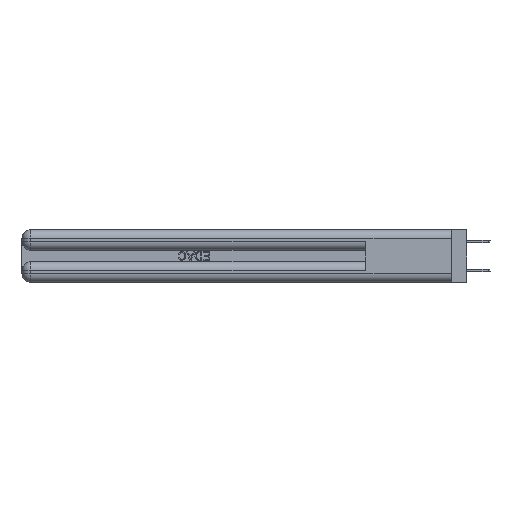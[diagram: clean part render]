
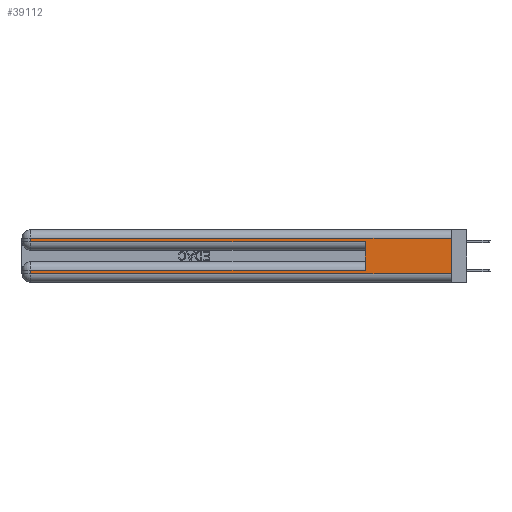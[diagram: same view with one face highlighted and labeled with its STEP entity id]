
A CAD part, left-side view. The second image highlights one B-rep face of the part: STEP entity #39112.
In plain terms, the highlighted planar face has unit normal (-1, 0, 0).
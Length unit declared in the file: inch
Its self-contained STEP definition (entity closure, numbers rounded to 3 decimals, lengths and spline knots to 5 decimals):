
#797 = CARTESIAN_POINT ( 'NONE',  ( 0., 0.6, 0.285 ) ) ;
#1355 = VECTOR ( 'NONE', #39381, 39.37008 ) ;
#1964 = VERTEX_POINT ( 'NONE', #797 ) ;
#2108 = EDGE_CURVE ( 'NONE', #13779, #41436, #46561, .T. ) ;
#2115 = EDGE_CURVE ( 'NONE', #35050, #1964, #35445, .T. ) ;
#3797 = CARTESIAN_POINT ( 'NONE',  ( 0., 2.94, 0.06 ) ) ;
#5570 = DIRECTION ( 'NONE',  ( 0., 0., 1. ) ) ;
#6320 = ORIENTED_EDGE ( 'NONE', *, *, #35680, .T. ) ;
#6403 = VECTOR ( 'NONE', #9231, 39.37008 ) ;
#6638 = PLANE ( 'NONE',  #15356 ) ;
#8556 = CARTESIAN_POINT ( 'NONE',  ( 0., 2.94, 0.31 ) ) ;
#9231 = DIRECTION ( 'NONE',  ( 0., 0., -1. ) ) ;
#9292 = ORIENTED_EDGE ( 'NONE', *, *, #16457, .F. ) ;
#9325 = DIRECTION ( 'NONE',  ( 0., 0., -1. ) ) ;
#10413 = ORIENTED_EDGE ( 'NONE', *, *, #24250, .T. ) ;
#10864 = VECTOR ( 'NONE', #22822, 39.37008 ) ;
#13252 = CARTESIAN_POINT ( 'NONE',  ( 0., 0., 0.285 ) ) ;
#13310 = CARTESIAN_POINT ( 'NONE',  ( 0., 0.6, 0.085 ) ) ;
#13517 = DIRECTION ( 'NONE',  ( 0., 0., -1. ) ) ;
#13779 = VERTEX_POINT ( 'NONE', #23196 ) ;
#14253 = DIRECTION ( 'NONE',  ( 0., 0., -1. ) ) ;
#15356 = AXIS2_PLACEMENT_3D ( 'NONE', #33063, #36834, #14253 ) ;
#16381 = EDGE_CURVE ( 'NONE', #35050, #13779, #21405, .T. ) ;
#16457 = EDGE_CURVE ( 'NONE', #17349, #16604, #37937, .T. ) ;
#16604 = VERTEX_POINT ( 'NONE', #18075 ) ;
#16807 = CARTESIAN_POINT ( 'NONE',  ( 0., 0., 0.085 ) ) ;
#16894 = CARTESIAN_POINT ( 'NONE',  ( 0., 2.94, 0.37 ) ) ;
#17349 = VERTEX_POINT ( 'NONE', #47285 ) ;
#18075 = CARTESIAN_POINT ( 'NONE',  ( 0., 0., 0.06 ) ) ;
#19204 = CARTESIAN_POINT ( 'NONE',  ( 0., 0., 0.31 ) ) ;
#19297 = VECTOR ( 'NONE', #9325, 39.37008 ) ;
#21405 = LINE ( 'NONE', #16807, #1355 ) ;
#22382 = LINE ( 'NONE', #13252, #34834 ) ;
#22822 = DIRECTION ( 'NONE',  ( 0., 1., 0. ) ) ;
#23196 = CARTESIAN_POINT ( 'NONE',  ( 0., 2.94, 0.085 ) ) ;
#24250 = EDGE_CURVE ( 'NONE', #41436, #16604, #29157, .T. ) ;
#25555 = EDGE_CURVE ( 'NONE', #47971, #45672, #38172, .T. ) ;
#27588 = ORIENTED_EDGE ( 'NONE', *, *, #16381, .T. ) ;
#28012 = CARTESIAN_POINT ( 'NONE',  ( 0., 2.94, 0.37 ) ) ;
#28179 = CARTESIAN_POINT ( 'NONE',  ( 0., 0.6, 0.145 ) ) ;
#29157 = LINE ( 'NONE', #39627, #47929 ) ;
#29270 = ORIENTED_EDGE ( 'NONE', *, *, #2108, .T. ) ;
#32113 = LINE ( 'NONE', #19204, #10864 ) ;
#32314 = CARTESIAN_POINT ( 'NONE',  ( 0., 0., 0.37 ) ) ;
#32898 = ORIENTED_EDGE ( 'NONE', *, *, #25555, .T. ) ;
#33063 = CARTESIAN_POINT ( 'NONE',  ( 0., 0., 0.37 ) ) ;
#34834 = VECTOR ( 'NONE', #39597, 39.37008 ) ;
#35050 = VERTEX_POINT ( 'NONE', #13310 ) ;
#35293 = EDGE_LOOP ( 'NONE', ( #9292, #39361, #32898, #6320, #36436, #27588, #29270, #10413 ) ) ;
#35445 = LINE ( 'NONE', #28179, #36602 ) ;
#35680 = EDGE_CURVE ( 'NONE', #45672, #1964, #22382, .T. ) ;
#36436 = ORIENTED_EDGE ( 'NONE', *, *, #2115, .F. ) ;
#36602 = VECTOR ( 'NONE', #5570, 39.37008 ) ;
#36834 = DIRECTION ( 'NONE',  ( 1., 0., 0. ) ) ;
#37937 = LINE ( 'NONE', #32314, #46714 ) ;
#38172 = LINE ( 'NONE', #16894, #19297 ) ;
#39112 = ADVANCED_FACE ( 'NONE', ( #43618 ), #6638, .F. ) ;
#39361 = ORIENTED_EDGE ( 'NONE', *, *, #43559, .T. ) ;
#39381 = DIRECTION ( 'NONE',  ( 0., 1., 0. ) ) ;
#39597 = DIRECTION ( 'NONE',  ( 0., -1., 0. ) ) ;
#39627 = CARTESIAN_POINT ( 'NONE',  ( 0., 0., 0.06 ) ) ;
#41436 = VERTEX_POINT ( 'NONE', #3797 ) ;
#43387 = DIRECTION ( 'NONE',  ( 0., -1., 0. ) ) ;
#43559 = EDGE_CURVE ( 'NONE', #17349, #47971, #32113, .T. ) ;
#43618 = FACE_OUTER_BOUND ( 'NONE', #35293, .T. ) ;
#45672 = VERTEX_POINT ( 'NONE', #47274 ) ;
#46561 = LINE ( 'NONE', #28012, #6403 ) ;
#46714 = VECTOR ( 'NONE', #13517, 39.37008 ) ;
#47274 = CARTESIAN_POINT ( 'NONE',  ( 0., 2.94, 0.285 ) ) ;
#47285 = CARTESIAN_POINT ( 'NONE',  ( 0., 0., 0.31 ) ) ;
#47929 = VECTOR ( 'NONE', #43387, 39.37008 ) ;
#47971 = VERTEX_POINT ( 'NONE', #8556 ) ;
